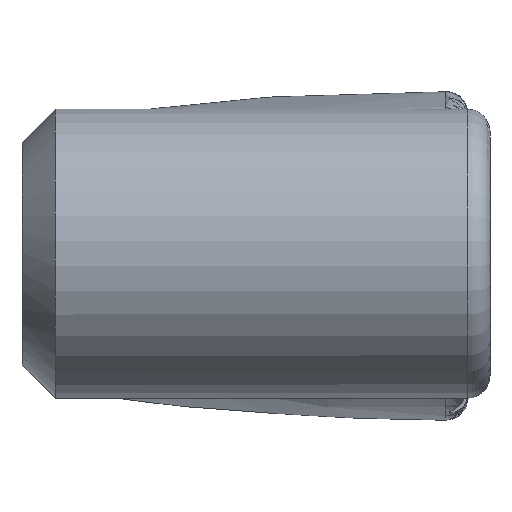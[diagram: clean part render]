
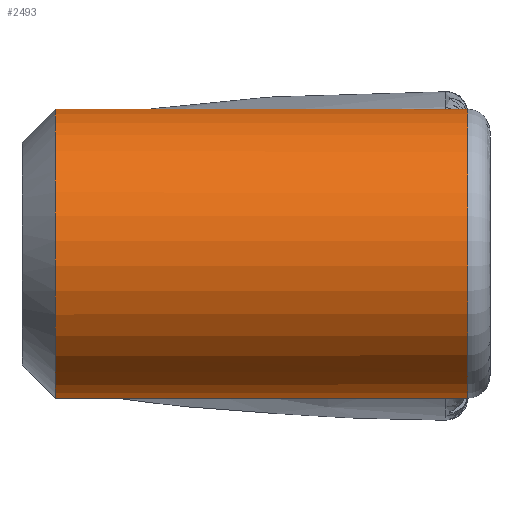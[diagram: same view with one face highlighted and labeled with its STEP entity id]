
A CAD part, top view. The second image highlights one B-rep face of the part: STEP entity #2493.
In plain terms, the highlighted cylindrical face has radius 6.5 mm (diameter 13 mm), a partial arc.
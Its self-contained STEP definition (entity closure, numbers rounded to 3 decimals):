
#45 = CARTESIAN_POINT ( 'NONE',  ( 79.815, 45.029, -26.587 ) ) ;
#52 = DIRECTION ( 'NONE',  ( -1., 0., 0. ) ) ;
#66 = ORIENTED_EDGE ( 'NONE', *, *, #6002, .T. ) ;
#68 = CARTESIAN_POINT ( 'NONE',  ( 80.556, 45.533, -26.803 ) ) ;
#289 = EDGE_CURVE ( 'NONE', #2129, #6281, #1277, .T. ) ;
#353 = CARTESIAN_POINT ( 'NONE',  ( 80.679, 49.629, -26.966 ) ) ;
#435 = CYLINDRICAL_SURFACE ( 'NONE', #2765, 6.5 ) ;
#481 = EDGE_LOOP ( 'NONE', ( #2937, #2103, #1713, #5421, #1407, #66 ) ) ;
#529 = LINE ( 'NONE', #3054, #5548 ) ;
#561 = DIRECTION ( 'NONE',  ( 1., 0., 0. ) ) ;
#569 = AXIS2_PLACEMENT_3D ( 'NONE', #4043, #6027, #1084 ) ;
#643 = DIRECTION ( 'NONE',  ( -1., 0., 0. ) ) ;
#996 = VERTEX_POINT ( 'NONE', #6269 ) ;
#1001 = EDGE_CURVE ( 'NONE', #6460, #996, #6024, .T. ) ;
#1038 = CARTESIAN_POINT ( 'NONE',  ( 80.304, 45.238, -26.683 ) ) ;
#1084 = DIRECTION ( 'NONE',  ( 0., 0., -1. ) ) ;
#1192 = FACE_OUTER_BOUND ( 'NONE', #481, .T. ) ;
#1277 = CIRCLE ( 'NONE', #569, 6.5 ) ;
#1340 = CARTESIAN_POINT ( 'NONE',  ( 80.304, 50.421, -26.683 ) ) ;
#1390 = CARTESIAN_POINT ( 'NONE',  ( 80.679, 49.761, -26.929 ) ) ;
#1407 = ORIENTED_EDGE ( 'NONE', *, *, #3846, .F. ) ;
#1412 = CARTESIAN_POINT ( 'NONE',  ( 79.816, 50.629, -26.587 ) ) ;
#1498 = CARTESIAN_POINT ( 'NONE',  ( 80.679, 49.629, -26.966 ) ) ;
#1525 = DIRECTION ( 'NONE',  ( 0., 0., -1. ) ) ;
#1544 = CARTESIAN_POINT ( 'NONE',  ( 80.653, 45.77, -26.887 ) ) ;
#1713 = ORIENTED_EDGE ( 'NONE', *, *, #6020, .F. ) ;
#1853 = CARTESIAN_POINT ( 'NONE',  ( 80.654, 49.888, -26.888 ) ) ;
#2103 = ORIENTED_EDGE ( 'NONE', *, *, #6315, .T. ) ;
#2129 = VERTEX_POINT ( 'NONE', #5214 ) ;
#2151 = B_SPLINE_CURVE_WITH_KNOTS ( 'NONE', 3,
 ( #6070, #45, #3545, #4041, #1038, #4555, #68, #1544, #4577, #5181 ),
 .UNSPECIFIED., .F., .F.,
 ( 4, 2, 2, 2, 4 ),
 ( 0., 0., 0.001, 0.001, 0.002 ),
 .UNSPECIFIED. ) ;
#2230 = LINE ( 'NONE', #5109, #2945 ) ;
#2254 = DIRECTION ( 'NONE',  ( 1., 0., 0. ) ) ;
#2493 = ADVANCED_FACE ( 'NONE', ( #1192 ), #435, .T. ) ;
#2572 = VERTEX_POINT ( 'NONE', #5518 ) ;
#2765 = AXIS2_PLACEMENT_3D ( 'NONE', #6076, #52, #1525 ) ;
#2937 = ORIENTED_EDGE ( 'NONE', *, *, #1001, .F. ) ;
#2945 = VECTOR ( 'NONE', #643, 1000. ) ;
#3054 = CARTESIAN_POINT ( 'NONE',  ( 75.679, 50.629, -26.587 ) ) ;
#3079 = B_SPLINE_CURVE_WITH_KNOTS ( 'NONE', 3,
 ( #353, #1390, #1853, #4345, #3884, #1340, #3412, #4414, #1412, #4867 ),
 .UNSPECIFIED., .F., .F.,
 ( 4, 2, 2, 2, 4 ),
 ( 0., 0., 0.001, 0.001, 0.002 ),
 .UNSPECIFIED. ) ;
#3220 = VERTEX_POINT ( 'NONE', #3952 ) ;
#3412 = CARTESIAN_POINT ( 'NONE',  ( 80.194, 50.497, -26.648 ) ) ;
#3545 = CARTESIAN_POINT ( 'NONE',  ( 79.949, 45.058, -26.6 ) ) ;
#3845 = CARTESIAN_POINT ( 'NONE',  ( 62.179, 45.029, -26.587 ) ) ;
#3846 = EDGE_CURVE ( 'NONE', #2572, #6281, #2230, .T. ) ;
#3884 = CARTESIAN_POINT ( 'NONE',  ( 80.485, 50.235, -26.76 ) ) ;
#3952 = CARTESIAN_POINT ( 'NONE',  ( 79.679, 50.629, -26.587 ) ) ;
#4041 = CARTESIAN_POINT ( 'NONE',  ( 80.194, 45.162, -26.648 ) ) ;
#4043 = CARTESIAN_POINT ( 'NONE',  ( 62.179, 47.829, -20.721 ) ) ;
#4274 = AXIS2_PLACEMENT_3D ( 'NONE', #5286, #2254, #5799 ) ;
#4345 = CARTESIAN_POINT ( 'NONE',  ( 80.556, 50.126, -26.803 ) ) ;
#4414 = CARTESIAN_POINT ( 'NONE',  ( 79.95, 50.601, -26.6 ) ) ;
#4555 = CARTESIAN_POINT ( 'NONE',  ( 80.484, 45.423, -26.76 ) ) ;
#4577 = CARTESIAN_POINT ( 'NONE',  ( 80.679, 45.898, -26.929 ) ) ;
#4867 = CARTESIAN_POINT ( 'NONE',  ( 79.679, 50.629, -26.587 ) ) ;
#5109 = CARTESIAN_POINT ( 'NONE',  ( 75.679, 45.029, -26.587 ) ) ;
#5181 = CARTESIAN_POINT ( 'NONE',  ( 80.679, 46.029, -26.966 ) ) ;
#5214 = CARTESIAN_POINT ( 'NONE',  ( 62.179, 50.629, -26.587 ) ) ;
#5286 = CARTESIAN_POINT ( 'NONE',  ( 80.679, 47.829, -20.721 ) ) ;
#5421 = ORIENTED_EDGE ( 'NONE', *, *, #289, .T. ) ;
#5518 = CARTESIAN_POINT ( 'NONE',  ( 79.679, 45.029, -26.587 ) ) ;
#5548 = VECTOR ( 'NONE', #561, 1000. ) ;
#5799 = DIRECTION ( 'NONE',  ( 0., 0., -1. ) ) ;
#6002 = EDGE_CURVE ( 'NONE', #2572, #996, #2151, .T. ) ;
#6020 = EDGE_CURVE ( 'NONE', #2129, #3220, #529, .T. ) ;
#6024 = CIRCLE ( 'NONE', #4274, 6.5 ) ;
#6027 = DIRECTION ( 'NONE',  ( 1., 0., 0. ) ) ;
#6070 = CARTESIAN_POINT ( 'NONE',  ( 79.679, 45.029, -26.587 ) ) ;
#6076 = CARTESIAN_POINT ( 'NONE',  ( 75.679, 47.829, -20.721 ) ) ;
#6269 = CARTESIAN_POINT ( 'NONE',  ( 80.679, 46.029, -26.966 ) ) ;
#6281 = VERTEX_POINT ( 'NONE', #3845 ) ;
#6315 = EDGE_CURVE ( 'NONE', #6460, #3220, #3079, .T. ) ;
#6460 = VERTEX_POINT ( 'NONE', #1498 ) ;
